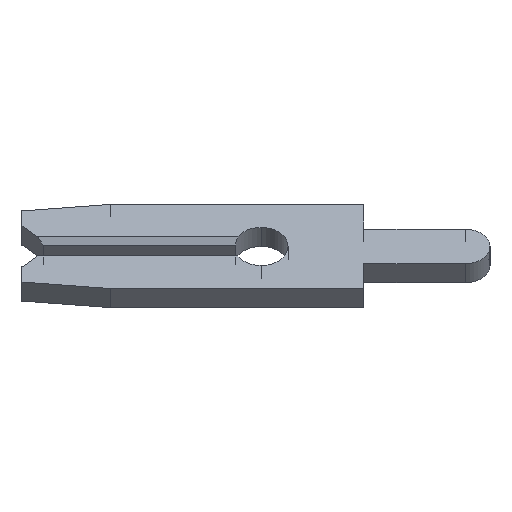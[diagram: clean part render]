
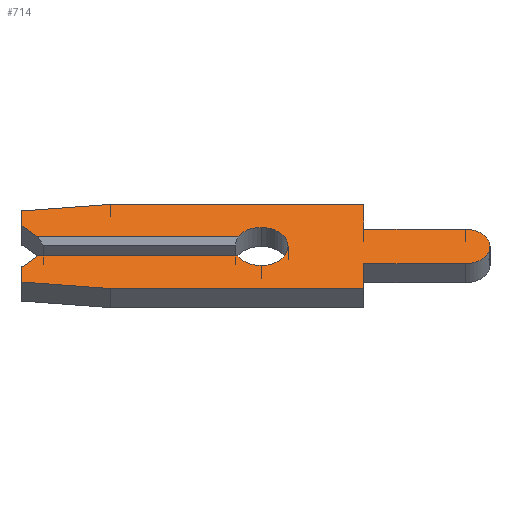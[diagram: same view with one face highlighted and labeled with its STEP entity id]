
A CAD part, left-side view. The second image highlights one B-rep face of the part: STEP entity #714.
In plain terms, the highlighted face is planar.
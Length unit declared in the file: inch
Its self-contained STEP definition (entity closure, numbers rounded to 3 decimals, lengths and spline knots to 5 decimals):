
#23 = CARTESIAN_POINT ( 'NONE',  ( -0.013, 0.231, -0.04857 ) ) ;
#31 = DIRECTION ( 'NONE',  ( 0., -1., 0. ) ) ;
#42 = VECTOR ( 'NONE', #1473, 39.37008 ) ;
#54 = CARTESIAN_POINT ( 'NONE',  ( -0.013, 0.216, 0.013 ) ) ;
#55 = VERTEX_POINT ( 'NONE', #939 ) ;
#59 = EDGE_CURVE ( 'NONE', #483, #703, #1076, .T. ) ;
#99 = PLANE ( 'NONE',  #348 ) ;
#103 = DIRECTION ( 'NONE',  ( 0., 0.707, 0.707 ) ) ;
#141 = VERTEX_POINT ( 'NONE', #23 ) ;
#145 = LINE ( 'NONE', #723, #930 ) ;
#147 = LINE ( 'NONE', #1437, #1334 ) ;
#152 = ORIENTED_EDGE ( 'NONE', *, *, #1752, .F. ) ;
#167 = VERTEX_POINT ( 'NONE', #526 ) ;
#196 = VECTOR ( 'NONE', #216, 39.37008 ) ;
#199 = CIRCLE ( 'NONE', #478, 0.026 ) ;
#205 = VECTOR ( 'NONE', #386, 39.37008 ) ;
#212 = LINE ( 'NONE', #910, #1910 ) ;
#216 = DIRECTION ( 'NONE',  ( 0., 0., -1. ) ) ;
#220 = CARTESIAN_POINT ( 'NONE',  ( -0.013, 0., -0.013 ) ) ;
#228 = EDGE_CURVE ( 'NONE', #1084, #55, #874, .T. ) ;
#239 = ORIENTED_EDGE ( 'NONE', *, *, #300, .F. ) ;
#241 = CARTESIAN_POINT ( 'NONE',  ( -0.013, 0., 0. ) ) ;
#247 = CARTESIAN_POINT ( 'NONE',  ( -0.013, 0.231, -0.028 ) ) ;
#252 = CARTESIAN_POINT ( 'NONE',  ( -0.013, 0.231, 0.04857 ) ) ;
#263 = VERTEX_POINT ( 'NONE', #972 ) ;
#271 = EDGE_CURVE ( 'NONE', #297, #141, #147, .T. ) ;
#276 = ORIENTED_EDGE ( 'NONE', *, *, #951, .F. ) ;
#297 = VERTEX_POINT ( 'NONE', #1579 ) ;
#300 = EDGE_CURVE ( 'NONE', #1043, #938, #1787, .T. ) ;
#331 = VERTEX_POINT ( 'NONE', #996 ) ;
#348 = AXIS2_PLACEMENT_3D ( 'NONE', #1177, #1006, #1315 ) ;
#363 = LINE ( 'NONE', #1837, #1741 ) ;
#378 = CARTESIAN_POINT ( 'NONE',  ( -0.013, -0.099, -0.0575 ) ) ;
#386 = DIRECTION ( 'NONE',  ( 0., 0., -1. ) ) ;
#387 = ORIENTED_EDGE ( 'NONE', *, *, #851, .F. ) ;
#397 = VECTOR ( 'NONE', #1303, 39.37008 ) ;
#399 = CARTESIAN_POINT ( 'NONE',  ( -0.013, -0.1975, 0.0235 ) ) ;
#421 = CIRCLE ( 'NONE', #917, 0.026 ) ;
#447 = DIRECTION ( 'NONE',  ( -1., 0., 0. ) ) ;
#453 = CIRCLE ( 'NONE', #1412, 0.0235 ) ;
#469 = VECTOR ( 'NONE', #1584, 39.37008 ) ;
#478 = AXIS2_PLACEMENT_3D ( 'NONE', #1498, #447, #1813 ) ;
#483 = VERTEX_POINT ( 'NONE', #54 ) ;
#526 = CARTESIAN_POINT ( 'NONE',  ( -0.013, -0.099, -0.0575 ) ) ;
#548 = EDGE_CURVE ( 'NONE', #938, #1106, #956, .T. ) ;
#562 = VERTEX_POINT ( 'NONE', #1774 ) ;
#570 = EDGE_CURVE ( 'NONE', #1106, #745, #978, .T. ) ;
#575 = ORIENTED_EDGE ( 'NONE', *, *, #725, .F. ) ;
#589 = CIRCLE ( 'NONE', #1738, 0.026 ) ;
#627 = VERTEX_POINT ( 'NONE', #247 ) ;
#629 = EDGE_CURVE ( 'NONE', #745, #1104, #453, .T. ) ;
#660 = VECTOR ( 'NONE', #1865, 39.37008 ) ;
#663 = LINE ( 'NONE', #1330, #1182 ) ;
#696 = DIRECTION ( 'NONE',  ( 0., 0.995, 0.105 ) ) ;
#698 = LINE ( 'NONE', #1658, #1029 ) ;
#703 = VERTEX_POINT ( 'NONE', #1928 ) ;
#707 = DIRECTION ( 'NONE',  ( 0., 1., 0. ) ) ;
#714 = ADVANCED_FACE ( 'NONE', ( #1089 ), #99, .F. ) ;
#723 = CARTESIAN_POINT ( 'NONE',  ( -0.013, -0.099, -0.0235 ) ) ;
#725 = EDGE_CURVE ( 'NONE', #841, #167, #1844, .T. ) ;
#736 = EDGE_LOOP ( 'NONE', ( #1954, #387, #918, #152, #1364, #1355, #1192, #1079, #276, #575, #1154, #837, #1071, #1456, #239, #1243, #893, #1959 ) ) ;
#745 = VERTEX_POINT ( 'NONE', #399 ) ;
#829 = EDGE_CURVE ( 'NONE', #263, #1268, #698, .T. ) ;
#837 = ORIENTED_EDGE ( 'NONE', *, *, #629, .F. ) ;
#841 = VERTEX_POINT ( 'NONE', #883 ) ;
#851 = EDGE_CURVE ( 'NONE', #331, #703, #199, .T. ) ;
#860 = EDGE_CURVE ( 'NONE', #483, #263, #212, .T. ) ;
#863 = DIRECTION ( 'NONE',  ( 1., 0., 0. ) ) ;
#874 = LINE ( 'NONE', #220, #469 ) ;
#883 = CARTESIAN_POINT ( 'NONE',  ( -0.013, -0.099, -0.0235 ) ) ;
#893 = ORIENTED_EDGE ( 'NONE', *, *, #829, .F. ) ;
#907 = CARTESIAN_POINT ( 'NONE',  ( -0.013, -0.099, 0.0575 ) ) ;
#910 = CARTESIAN_POINT ( 'NONE',  ( -0.013, 0.2105, 0.0075 ) ) ;
#917 = AXIS2_PLACEMENT_3D ( 'NONE', #241, #1032, #1486 ) ;
#918 = ORIENTED_EDGE ( 'NONE', *, *, #1578, .F. ) ;
#930 = VECTOR ( 'NONE', #707, 39.37008 ) ;
#938 = VERTEX_POINT ( 'NONE', #907 ) ;
#939 = CARTESIAN_POINT ( 'NONE',  ( -0.013, 0.02252, -0.013 ) ) ;
#951 = EDGE_CURVE ( 'NONE', #167, #297, #1155, .T. ) ;
#956 = LINE ( 'NONE', #980, #196 ) ;
#972 = CARTESIAN_POINT ( 'NONE',  ( -0.013, 0.231, 0.028 ) ) ;
#978 = LINE ( 'NONE', #1331, #397 ) ;
#980 = CARTESIAN_POINT ( 'NONE',  ( -0.013, -0.099, 0.0575 ) ) ;
#995 = CARTESIAN_POINT ( 'NONE',  ( -0.013, 0., 0. ) ) ;
#996 = CARTESIAN_POINT ( 'NONE',  ( -0.013, 0., 0.026 ) ) ;
#1005 = DIRECTION ( 'NONE',  ( 0., -0.707, 0.707 ) ) ;
#1006 = DIRECTION ( 'NONE',  ( 1., 0., 0. ) ) ;
#1015 = DIRECTION ( 'NONE',  ( 0., 0., 1. ) ) ;
#1029 = VECTOR ( 'NONE', #1188, 39.37008 ) ;
#1032 = DIRECTION ( 'NONE',  ( -1., 0., 0. ) ) ;
#1038 = EDGE_CURVE ( 'NONE', #1268, #1043, #1165, .T. ) ;
#1043 = VERTEX_POINT ( 'NONE', #1058 ) ;
#1058 = CARTESIAN_POINT ( 'NONE',  ( -0.013, 0.146, 0.0575 ) ) ;
#1071 = ORIENTED_EDGE ( 'NONE', *, *, #570, .F. ) ;
#1076 = LINE ( 'NONE', #1114, #660 ) ;
#1079 = ORIENTED_EDGE ( 'NONE', *, *, #271, .F. ) ;
#1084 = VERTEX_POINT ( 'NONE', #1538 ) ;
#1089 = FACE_OUTER_BOUND ( 'NONE', #736, .T. ) ;
#1104 = VERTEX_POINT ( 'NONE', #1541 ) ;
#1106 = VERTEX_POINT ( 'NONE', #1241 ) ;
#1114 = CARTESIAN_POINT ( 'NONE',  ( -0.013, 0.231, 0.013 ) ) ;
#1131 = DIRECTION ( 'NONE',  ( 0., 0., -1. ) ) ;
#1154 = ORIENTED_EDGE ( 'NONE', *, *, #1777, .F. ) ;
#1155 = LINE ( 'NONE', #1454, #42 ) ;
#1165 = LINE ( 'NONE', #252, #1769 ) ;
#1177 = CARTESIAN_POINT ( 'NONE',  ( -0.013, 0., 0. ) ) ;
#1182 = VECTOR ( 'NONE', #1005, 39.37008 ) ;
#1188 = DIRECTION ( 'NONE',  ( 0., 0., 1. ) ) ;
#1192 = ORIENTED_EDGE ( 'NONE', *, *, #1199, .F. ) ;
#1199 = EDGE_CURVE ( 'NONE', #141, #627, #363, .T. ) ;
#1236 = CARTESIAN_POINT ( 'NONE',  ( -0.013, 0.231, 0.04857 ) ) ;
#1241 = CARTESIAN_POINT ( 'NONE',  ( -0.013, -0.099, 0.0235 ) ) ;
#1243 = ORIENTED_EDGE ( 'NONE', *, *, #1038, .F. ) ;
#1268 = VERTEX_POINT ( 'NONE', #1236 ) ;
#1303 = DIRECTION ( 'NONE',  ( 0., -1., 0. ) ) ;
#1315 = DIRECTION ( 'NONE',  ( 0., 0., -1. ) ) ;
#1330 = CARTESIAN_POINT ( 'NONE',  ( -0.013, 0.2105, -0.0075 ) ) ;
#1331 = CARTESIAN_POINT ( 'NONE',  ( -0.013, -0.099, 0.0235 ) ) ;
#1334 = VECTOR ( 'NONE', #696, 39.37008 ) ;
#1336 = DIRECTION ( 'NONE',  ( 0., -0.995, 0.105 ) ) ;
#1355 = ORIENTED_EDGE ( 'NONE', *, *, #1724, .F. ) ;
#1364 = ORIENTED_EDGE ( 'NONE', *, *, #228, .F. ) ;
#1367 = DIRECTION ( 'NONE',  ( 0., 0., 1. ) ) ;
#1382 = VECTOR ( 'NONE', #31, 39.37008 ) ;
#1412 = AXIS2_PLACEMENT_3D ( 'NONE', #1466, #863, #1015 ) ;
#1437 = CARTESIAN_POINT ( 'NONE',  ( -0.013, 0.231, -0.04857 ) ) ;
#1454 = CARTESIAN_POINT ( 'NONE',  ( -0.013, 0.146, -0.0575 ) ) ;
#1456 = ORIENTED_EDGE ( 'NONE', *, *, #548, .F. ) ;
#1466 = CARTESIAN_POINT ( 'NONE',  ( -0.013, -0.1975, 0. ) ) ;
#1473 = DIRECTION ( 'NONE',  ( 0., 1., 0. ) ) ;
#1486 = DIRECTION ( 'NONE',  ( 0., 0., -1. ) ) ;
#1498 = CARTESIAN_POINT ( 'NONE',  ( -0.013, 0., 0. ) ) ;
#1538 = CARTESIAN_POINT ( 'NONE',  ( -0.013, 0.216, -0.013 ) ) ;
#1541 = CARTESIAN_POINT ( 'NONE',  ( -0.013, -0.1975, -0.0235 ) ) ;
#1578 = EDGE_CURVE ( 'NONE', #562, #331, #589, .T. ) ;
#1579 = CARTESIAN_POINT ( 'NONE',  ( -0.013, 0.146, -0.0575 ) ) ;
#1584 = DIRECTION ( 'NONE',  ( 0., -1., 0. ) ) ;
#1658 = CARTESIAN_POINT ( 'NONE',  ( -0.013, 0.231, 0.028 ) ) ;
#1724 = EDGE_CURVE ( 'NONE', #627, #1084, #663, .T. ) ;
#1738 = AXIS2_PLACEMENT_3D ( 'NONE', #995, #1898, #1131 ) ;
#1741 = VECTOR ( 'NONE', #1367, 39.37008 ) ;
#1752 = EDGE_CURVE ( 'NONE', #55, #562, #421, .T. ) ;
#1769 = VECTOR ( 'NONE', #1336, 39.37008 ) ;
#1774 = CARTESIAN_POINT ( 'NONE',  ( -0.013, 0., -0.026 ) ) ;
#1777 = EDGE_CURVE ( 'NONE', #1104, #841, #145, .T. ) ;
#1787 = LINE ( 'NONE', #1890, #1382 ) ;
#1813 = DIRECTION ( 'NONE',  ( 0., 0., -1. ) ) ;
#1837 = CARTESIAN_POINT ( 'NONE',  ( -0.013, 0.231, -0.028 ) ) ;
#1844 = LINE ( 'NONE', #378, #205 ) ;
#1865 = DIRECTION ( 'NONE',  ( 0., -1., 0. ) ) ;
#1890 = CARTESIAN_POINT ( 'NONE',  ( -0.013, 0.146, 0.0575 ) ) ;
#1898 = DIRECTION ( 'NONE',  ( -1., 0., 0. ) ) ;
#1910 = VECTOR ( 'NONE', #103, 39.37008 ) ;
#1928 = CARTESIAN_POINT ( 'NONE',  ( -0.013, 0.02252, 0.013 ) ) ;
#1954 = ORIENTED_EDGE ( 'NONE', *, *, #59, .T. ) ;
#1959 = ORIENTED_EDGE ( 'NONE', *, *, #860, .F. ) ;
